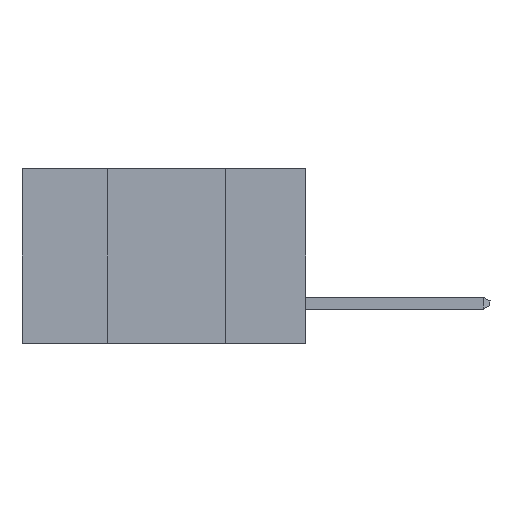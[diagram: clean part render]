
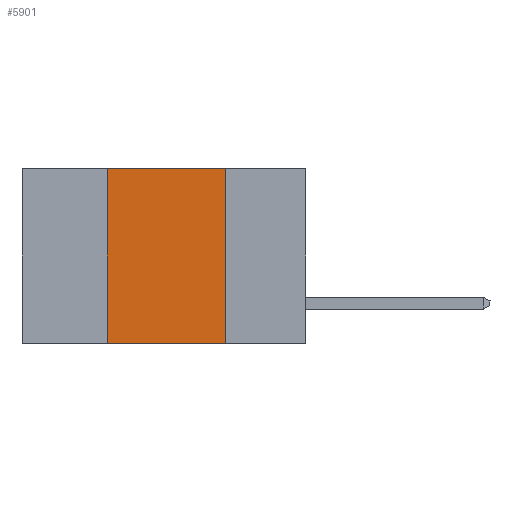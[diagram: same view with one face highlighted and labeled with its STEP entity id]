
A CAD part, left-side view. The second image highlights one B-rep face of the part: STEP entity #5901.
In plain terms, the highlighted planar face has unit normal (-1, 0, 0).
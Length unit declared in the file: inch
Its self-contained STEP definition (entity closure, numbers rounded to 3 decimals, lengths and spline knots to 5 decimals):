
#96 = VERTEX_POINT ( 'NONE', #8527 ) ;
#174 = CARTESIAN_POINT ( 'NONE',  ( 0., 0.17, 0. ) ) ;
#777 = VERTEX_POINT ( 'NONE', #1138 ) ;
#1138 = CARTESIAN_POINT ( 'NONE',  ( 0., 0.17, -0.37 ) ) ;
#1224 = ORIENTED_EDGE ( 'NONE', *, *, #2554, .F. ) ;
#1225 = VECTOR ( 'NONE', #5187, 39.37008 ) ;
#1276 = VECTOR ( 'NONE', #8534, 39.37008 ) ;
#1925 = CARTESIAN_POINT ( 'NONE',  ( 0., 0.6, 0. ) ) ;
#2454 = LINE ( 'NONE', #5244, #8210 ) ;
#2537 = CARTESIAN_POINT ( 'NONE',  ( 0., 0.6, 0. ) ) ;
#2554 = EDGE_CURVE ( 'NONE', #96, #3288, #2454, .T. ) ;
#2714 = VECTOR ( 'NONE', #3744, 39.37008 ) ;
#3288 = VERTEX_POINT ( 'NONE', #5394 ) ;
#3459 = ORIENTED_EDGE ( 'NONE', *, *, #10177, .F. ) ;
#3633 = DIRECTION ( 'NONE',  ( 0., 0., -1. ) ) ;
#3744 = DIRECTION ( 'NONE',  ( 0., 0., -1. ) ) ;
#3930 = FACE_OUTER_BOUND ( 'NONE', #10933, .T. ) ;
#5156 = LINE ( 'NONE', #6353, #2714 ) ;
#5187 = DIRECTION ( 'NONE',  ( 0., -1., 0. ) ) ;
#5244 = CARTESIAN_POINT ( 'NONE',  ( 0., 0.42, 0. ) ) ;
#5394 = CARTESIAN_POINT ( 'NONE',  ( 0., 0.42, 0. ) ) ;
#5519 = AXIS2_PLACEMENT_3D ( 'NONE', #1925, #7939, #3633 ) ;
#5621 = ORIENTED_EDGE ( 'NONE', *, *, #7728, .T. ) ;
#5675 = LINE ( 'NONE', #11085, #1225 ) ;
#5901 = ADVANCED_FACE ( 'NONE', ( #3930 ), #8075, .F. ) ;
#6353 = CARTESIAN_POINT ( 'NONE',  ( 0., 0.17, 0. ) ) ;
#6751 = VERTEX_POINT ( 'NONE', #174 ) ;
#6774 = LINE ( 'NONE', #2537, #1276 ) ;
#6885 = EDGE_CURVE ( 'NONE', #6751, #777, #5156, .T. ) ;
#7412 = ORIENTED_EDGE ( 'NONE', *, *, #6885, .F. ) ;
#7728 = EDGE_CURVE ( 'NONE', #96, #777, #5675, .T. ) ;
#7939 = DIRECTION ( 'NONE',  ( 1., 0., 0. ) ) ;
#8075 = PLANE ( 'NONE',  #5519 ) ;
#8210 = VECTOR ( 'NONE', #9529, 39.37008 ) ;
#8527 = CARTESIAN_POINT ( 'NONE',  ( 0., 0.42, -0.37 ) ) ;
#8534 = DIRECTION ( 'NONE',  ( 0., -1., 0. ) ) ;
#9529 = DIRECTION ( 'NONE',  ( 0., 0., 1. ) ) ;
#10177 = EDGE_CURVE ( 'NONE', #3288, #6751, #6774, .T. ) ;
#10933 = EDGE_LOOP ( 'NONE', ( #7412, #3459, #1224, #5621 ) ) ;
#11085 = CARTESIAN_POINT ( 'NONE',  ( 0., 0.6, -0.37 ) ) ;
